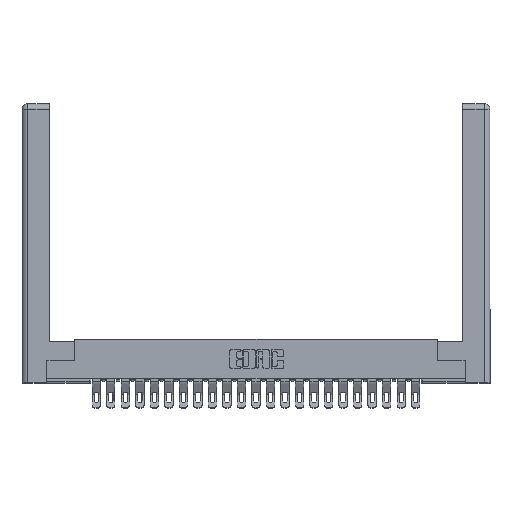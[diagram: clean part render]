
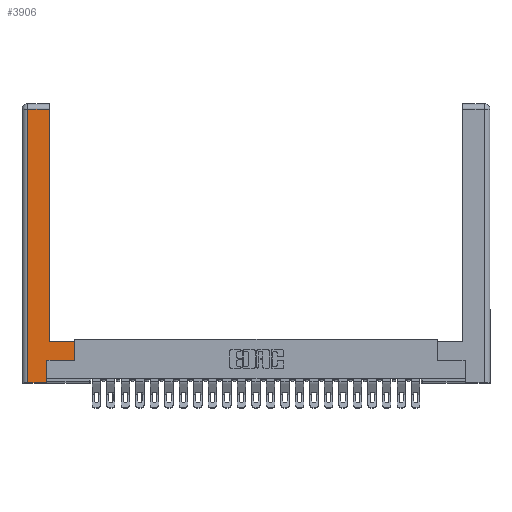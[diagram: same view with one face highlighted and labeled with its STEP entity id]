
A CAD part, top view. The second image highlights one B-rep face of the part: STEP entity #3906.
In plain terms, the highlighted planar face has unit normal (0, 0, 1).
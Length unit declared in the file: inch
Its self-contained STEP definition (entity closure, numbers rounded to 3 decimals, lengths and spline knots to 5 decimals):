
#741 = VECTOR ( 'NONE', #2198, 39.37008 ) ;
#752 = CARTESIAN_POINT ( 'NONE',  ( 0.265, 0., 0. ) ) ;
#777 = VERTEX_POINT ( 'NONE', #1477 ) ;
#961 = PLANE ( 'NONE',  #3724 ) ;
#1340 = VERTEX_POINT ( 'NONE', #4540 ) ;
#1452 = VECTOR ( 'NONE', #13971, 39.37008 ) ;
#1477 = CARTESIAN_POINT ( 'NONE',  ( 0.565, 0.45, 0. ) ) ;
#1533 = ORIENTED_EDGE ( 'NONE', *, *, #1609, .T. ) ;
#1609 = EDGE_CURVE ( 'NONE', #21921, #17738, #4311, .T. ) ;
#2057 = VECTOR ( 'NONE', #10551, 39.37008 ) ;
#2176 = DIRECTION ( 'NONE',  ( -1., 0., 0. ) ) ;
#2195 = EDGE_CURVE ( 'NONE', #17738, #18815, #23417, .T. ) ;
#2198 = DIRECTION ( 'NONE',  ( 0., 1., 0. ) ) ;
#2654 = VERTEX_POINT ( 'NONE', #13396 ) ;
#3050 = VECTOR ( 'NONE', #17202, 39.37008 ) ;
#3536 = DIRECTION ( 'NONE',  ( 1., 0., 0. ) ) ;
#3705 = ORIENTED_EDGE ( 'NONE', *, *, #2195, .T. ) ;
#3724 = AXIS2_PLACEMENT_3D ( 'NONE', #9029, #22777, #14983 ) ;
#3906 = ADVANCED_FACE ( 'NONE', ( #7646 ), #961, .F. ) ;
#3913 = ORIENTED_EDGE ( 'NONE', *, *, #4147, .T. ) ;
#4147 = EDGE_CURVE ( 'NONE', #4443, #777, #24884, .T. ) ;
#4202 = CARTESIAN_POINT ( 'NONE',  ( 0.295, 0.45, 0. ) ) ;
#4285 = EDGE_CURVE ( 'NONE', #777, #21921, #20771, .T. ) ;
#4311 = LINE ( 'NONE', #15973, #1452 ) ;
#4443 = VERTEX_POINT ( 'NONE', #12481 ) ;
#4540 = CARTESIAN_POINT ( 'NONE',  ( 0.265, 0., 0. ) ) ;
#5448 = LINE ( 'NONE', #20127, #741 ) ;
#5538 = CARTESIAN_POINT ( 'NONE',  ( 0.0615, 2.94, 0. ) ) ;
#6021 = EDGE_CURVE ( 'NONE', #19101, #1340, #25921, .T. ) ;
#6685 = CARTESIAN_POINT ( 'NONE',  ( 0.295, 0.45, 0. ) ) ;
#7325 = VECTOR ( 'NONE', #17766, 39.37008 ) ;
#7415 = ORIENTED_EDGE ( 'NONE', *, *, #6021, .T. ) ;
#7646 = FACE_OUTER_BOUND ( 'NONE', #8175, .T. ) ;
#7803 = EDGE_CURVE ( 'NONE', #2654, #4443, #22356, .T. ) ;
#7889 = CARTESIAN_POINT ( 'NONE',  ( 0.565, 0.45, 0. ) ) ;
#8086 = DIRECTION ( 'NONE',  ( -1., 0., 0. ) ) ;
#8175 = EDGE_LOOP ( 'NONE', ( #1533, #3705, #14205, #7415, #10685, #11982, #3913, #11436 ) ) ;
#9029 = CARTESIAN_POINT ( 'NONE',  ( 0., 0., 0. ) ) ;
#9326 = LINE ( 'NONE', #25219, #3050 ) ;
#10149 = CARTESIAN_POINT ( 'NONE',  ( 0.0615, 0., 0. ) ) ;
#10551 = DIRECTION ( 'NONE',  ( 1., 0., 0. ) ) ;
#10685 = ORIENTED_EDGE ( 'NONE', *, *, #20973, .T. ) ;
#11436 = ORIENTED_EDGE ( 'NONE', *, *, #4285, .T. ) ;
#11982 = ORIENTED_EDGE ( 'NONE', *, *, #7803, .T. ) ;
#12292 = VECTOR ( 'NONE', #2176, 39.37008 ) ;
#12481 = CARTESIAN_POINT ( 'NONE',  ( 0.565, 0.245, 0. ) ) ;
#13396 = CARTESIAN_POINT ( 'NONE',  ( 0.265, 0.245, 0. ) ) ;
#13971 = DIRECTION ( 'NONE',  ( 0., 1., 0. ) ) ;
#14205 = ORIENTED_EDGE ( 'NONE', *, *, #18050, .T. ) ;
#14983 = DIRECTION ( 'NONE',  ( -1., 0., 0. ) ) ;
#15355 = CARTESIAN_POINT ( 'NONE',  ( 0.0615, 2.94, 0. ) ) ;
#15973 = CARTESIAN_POINT ( 'NONE',  ( 0.295, 3., 0. ) ) ;
#17023 = VECTOR ( 'NONE', #3536, 39.37008 ) ;
#17202 = DIRECTION ( 'NONE',  ( 0., -1., 0. ) ) ;
#17738 = VERTEX_POINT ( 'NONE', #22702 ) ;
#17762 = VECTOR ( 'NONE', #8086, 39.37008 ) ;
#17766 = DIRECTION ( 'NONE',  ( 0., 1., 0. ) ) ;
#18050 = EDGE_CURVE ( 'NONE', #18815, #19101, #9326, .T. ) ;
#18815 = VERTEX_POINT ( 'NONE', #15355 ) ;
#19101 = VERTEX_POINT ( 'NONE', #10149 ) ;
#20127 = CARTESIAN_POINT ( 'NONE',  ( 0.265, 0.245, 0. ) ) ;
#20771 = LINE ( 'NONE', #4202, #12292 ) ;
#20973 = EDGE_CURVE ( 'NONE', #1340, #2654, #5448, .T. ) ;
#21732 = CARTESIAN_POINT ( 'NONE',  ( 0.565, 0.245, 0. ) ) ;
#21921 = VERTEX_POINT ( 'NONE', #6685 ) ;
#22356 = LINE ( 'NONE', #21732, #17023 ) ;
#22702 = CARTESIAN_POINT ( 'NONE',  ( 0.295, 2.94, 0. ) ) ;
#22777 = DIRECTION ( 'NONE',  ( 0., 0., -1. ) ) ;
#23417 = LINE ( 'NONE', #5538, #17762 ) ;
#24884 = LINE ( 'NONE', #7889, #7325 ) ;
#25219 = CARTESIAN_POINT ( 'NONE',  ( 0.0615, 0., 0. ) ) ;
#25921 = LINE ( 'NONE', #752, #2057 ) ;
